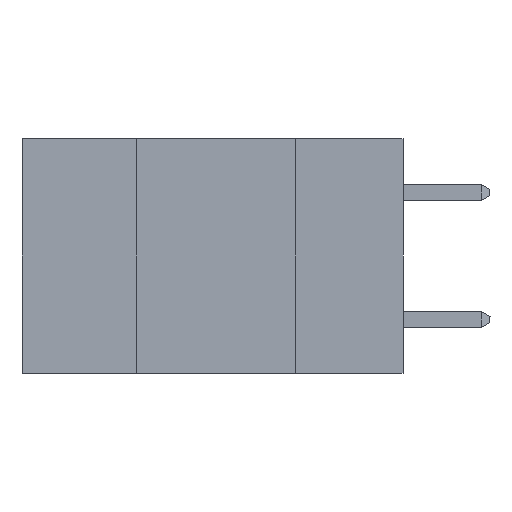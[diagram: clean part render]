
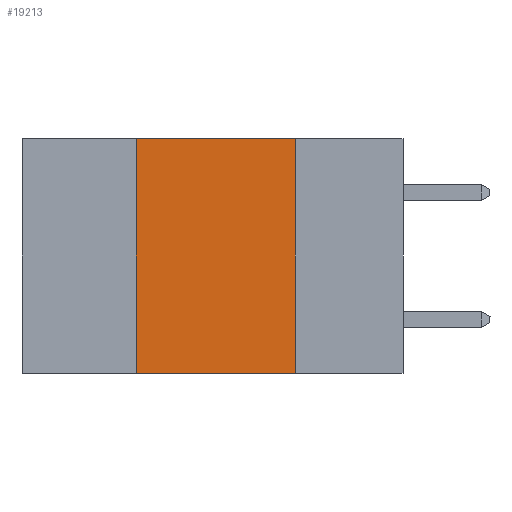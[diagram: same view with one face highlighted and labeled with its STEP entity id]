
A CAD part, left-side view. The second image highlights one B-rep face of the part: STEP entity #19213.
In plain terms, the highlighted planar face has unit normal (-1, 0, 0).
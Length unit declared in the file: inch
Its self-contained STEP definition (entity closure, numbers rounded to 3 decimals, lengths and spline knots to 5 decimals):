
#407 = ORIENTED_EDGE ( 'NONE', *, *, #33037, .F. ) ;
#2033 = CARTESIAN_POINT ( 'NONE',  ( 0., 0.6, 0. ) ) ;
#4638 = CARTESIAN_POINT ( 'NONE',  ( 0., 0.42, -0.37 ) ) ;
#7763 = VERTEX_POINT ( 'NONE', #29989 ) ;
#8709 = DIRECTION ( 'NONE',  ( 0., 0., -1. ) ) ;
#11132 = CARTESIAN_POINT ( 'NONE',  ( 0., 0.42, 0. ) ) ;
#13831 = VERTEX_POINT ( 'NONE', #37113 ) ;
#16267 = LINE ( 'NONE', #2033, #37597 ) ;
#18676 = CARTESIAN_POINT ( 'NONE',  ( 0., 0.6, 0. ) ) ;
#19213 = ADVANCED_FACE ( 'NONE', ( #42833 ), #35841, .F. ) ;
#20164 = LINE ( 'NONE', #34156, #35302 ) ;
#20773 = VERTEX_POINT ( 'NONE', #4638 ) ;
#22794 = ORIENTED_EDGE ( 'NONE', *, *, #30711, .F. ) ;
#23194 = EDGE_CURVE ( 'NONE', #13831, #40031, #16267, .T. ) ;
#26307 = CARTESIAN_POINT ( 'NONE',  ( 0., 0.6, -0.37 ) ) ;
#27375 = DIRECTION ( 'NONE',  ( 0., 0., -1. ) ) ;
#28084 = DIRECTION ( 'NONE',  ( 0., 0., 1. ) ) ;
#28632 = DIRECTION ( 'NONE',  ( 0., -1., 0. ) ) ;
#29586 = DIRECTION ( 'NONE',  ( 0., -1., 0. ) ) ;
#29989 = CARTESIAN_POINT ( 'NONE',  ( 0., 0.17, -0.37 ) ) ;
#30425 = EDGE_CURVE ( 'NONE', #20773, #7763, #36472, .T. ) ;
#30711 = EDGE_CURVE ( 'NONE', #20773, #13831, #32123, .T. ) ;
#30964 = AXIS2_PLACEMENT_3D ( 'NONE', #18676, #32205, #8709 ) ;
#31500 = ORIENTED_EDGE ( 'NONE', *, *, #23194, .F. ) ;
#32123 = LINE ( 'NONE', #11132, #33715 ) ;
#32205 = DIRECTION ( 'NONE',  ( 1., 0., 0. ) ) ;
#33037 = EDGE_CURVE ( 'NONE', #40031, #7763, #20164, .T. ) ;
#33715 = VECTOR ( 'NONE', #28084, 39.37008 ) ;
#34156 = CARTESIAN_POINT ( 'NONE',  ( 0., 0.17, 0. ) ) ;
#34329 = ORIENTED_EDGE ( 'NONE', *, *, #30425, .T. ) ;
#34698 = CARTESIAN_POINT ( 'NONE',  ( 0., 0.17, 0. ) ) ;
#35302 = VECTOR ( 'NONE', #27375, 39.37008 ) ;
#35841 = PLANE ( 'NONE',  #30964 ) ;
#35918 = VECTOR ( 'NONE', #28632, 39.37008 ) ;
#36472 = LINE ( 'NONE', #26307, #35918 ) ;
#37113 = CARTESIAN_POINT ( 'NONE',  ( 0., 0.42, 0. ) ) ;
#37597 = VECTOR ( 'NONE', #29586, 39.37008 ) ;
#38139 = EDGE_LOOP ( 'NONE', ( #407, #31500, #22794, #34329 ) ) ;
#40031 = VERTEX_POINT ( 'NONE', #34698 ) ;
#42833 = FACE_OUTER_BOUND ( 'NONE', #38139, .T. ) ;
